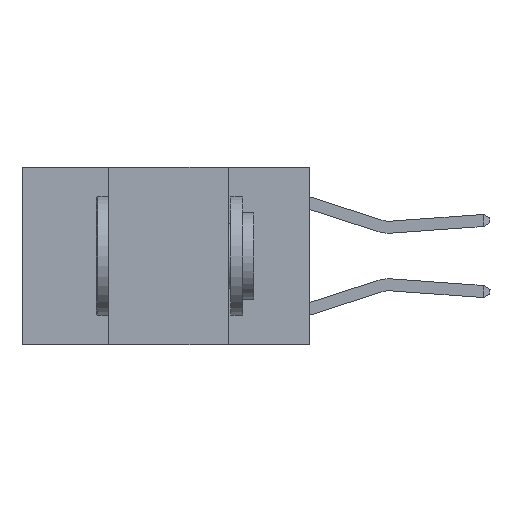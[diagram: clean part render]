
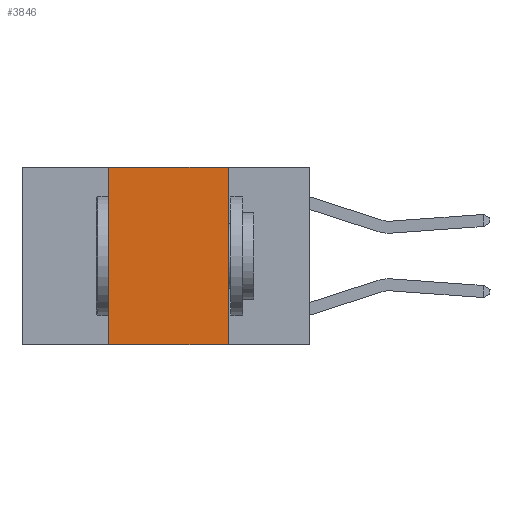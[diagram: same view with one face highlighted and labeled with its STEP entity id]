
A CAD part, left-side view. The second image highlights one B-rep face of the part: STEP entity #3846.
In plain terms, the highlighted planar face has unit normal (-1, 0, 0).
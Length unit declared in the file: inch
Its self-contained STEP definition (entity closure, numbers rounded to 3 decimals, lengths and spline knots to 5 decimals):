
#1 = ORIENTED_EDGE ( 'NONE', *, *, #1595, .F. ) ;
#36 = DIRECTION ( 'NONE',  ( 0., 0., 1. ) ) ;
#358 = ORIENTED_EDGE ( 'NONE', *, *, #817, .F. ) ;
#817 = EDGE_CURVE ( 'NONE', #11298, #2219, #13411, .T. ) ;
#1595 = EDGE_CURVE ( 'NONE', #13262, #5005, #7853, .T. ) ;
#2219 = VERTEX_POINT ( 'NONE', #2513 ) ;
#2513 = CARTESIAN_POINT ( 'NONE',  ( 0., 0.42, 0. ) ) ;
#2719 = LINE ( 'NONE', #3467, #8795 ) ;
#3069 = CARTESIAN_POINT ( 'NONE',  ( 0., 0.17, 0. ) ) ;
#3341 = DIRECTION ( 'NONE',  ( 1., 0., 0. ) ) ;
#3467 = CARTESIAN_POINT ( 'NONE',  ( 0., 0.6, 0. ) ) ;
#3747 = EDGE_CURVE ( 'NONE', #11298, #5005, #8636, .T. ) ;
#3846 = ADVANCED_FACE ( 'NONE', ( #5274 ), #8176, .F. ) ;
#4069 = CARTESIAN_POINT ( 'NONE',  ( 0., 0.42, -0.37 ) ) ;
#4297 = EDGE_CURVE ( 'NONE', #2219, #13262, #2719, .T. ) ;
#4725 = VECTOR ( 'NONE', #5178, 39.37008 ) ;
#5005 = VERTEX_POINT ( 'NONE', #15083 ) ;
#5064 = VECTOR ( 'NONE', #9979, 39.37008 ) ;
#5140 = CARTESIAN_POINT ( 'NONE',  ( 0., 0.6, -0.37 ) ) ;
#5178 = DIRECTION ( 'NONE',  ( 0., -1., 0. ) ) ;
#5274 = FACE_OUTER_BOUND ( 'NONE', #8859, .T. ) ;
#5961 = DIRECTION ( 'NONE',  ( 0., -1., 0. ) ) ;
#7687 = CARTESIAN_POINT ( 'NONE',  ( 0., 0.42, 0. ) ) ;
#7853 = LINE ( 'NONE', #10064, #5064 ) ;
#8176 = PLANE ( 'NONE',  #8879 ) ;
#8636 = LINE ( 'NONE', #5140, #4725 ) ;
#8795 = VECTOR ( 'NONE', #5961, 39.37008 ) ;
#8859 = EDGE_LOOP ( 'NONE', ( #1, #9596, #358, #9984 ) ) ;
#8879 = AXIS2_PLACEMENT_3D ( 'NONE', #10592, #3341, #11751 ) ;
#9570 = VECTOR ( 'NONE', #36, 39.37008 ) ;
#9596 = ORIENTED_EDGE ( 'NONE', *, *, #4297, .F. ) ;
#9979 = DIRECTION ( 'NONE',  ( 0., 0., -1. ) ) ;
#9984 = ORIENTED_EDGE ( 'NONE', *, *, #3747, .T. ) ;
#10064 = CARTESIAN_POINT ( 'NONE',  ( 0., 0.17, 0. ) ) ;
#10592 = CARTESIAN_POINT ( 'NONE',  ( 0., 0.6, 0. ) ) ;
#11298 = VERTEX_POINT ( 'NONE', #4069 ) ;
#11751 = DIRECTION ( 'NONE',  ( 0., 0., -1. ) ) ;
#13262 = VERTEX_POINT ( 'NONE', #3069 ) ;
#13411 = LINE ( 'NONE', #7687, #9570 ) ;
#15083 = CARTESIAN_POINT ( 'NONE',  ( 0., 0.17, -0.37 ) ) ;
